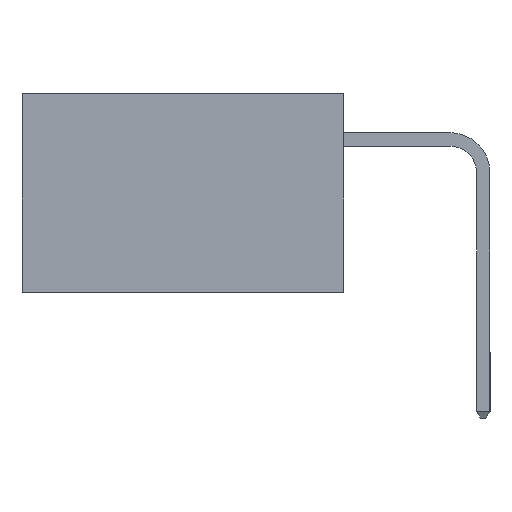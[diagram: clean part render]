
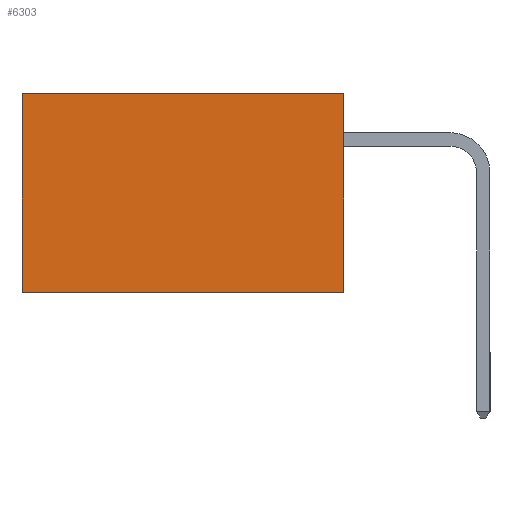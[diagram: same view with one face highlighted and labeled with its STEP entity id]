
A CAD part, left-side view. The second image highlights one B-rep face of the part: STEP entity #6303.
In plain terms, the highlighted planar face has unit normal (-1, 0, 0).
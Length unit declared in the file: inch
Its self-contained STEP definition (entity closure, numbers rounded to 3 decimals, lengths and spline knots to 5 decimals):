
#515 = VERTEX_POINT ( 'NONE', #8125 ) ;
#1023 = VECTOR ( 'NONE', #13386, 39.37008 ) ;
#2256 = VERTEX_POINT ( 'NONE', #5713 ) ;
#2532 = VERTEX_POINT ( 'NONE', #4521 ) ;
#2744 = FACE_OUTER_BOUND ( 'NONE', #3717, .T. ) ;
#2835 = ORIENTED_EDGE ( 'NONE', *, *, #6793, .T. ) ;
#2993 = ORIENTED_EDGE ( 'NONE', *, *, #3714, .T. ) ;
#3466 = EDGE_CURVE ( 'NONE', #515, #2256, #14345, .T. ) ;
#3616 = ORIENTED_EDGE ( 'NONE', *, *, #3466, .F. ) ;
#3714 = EDGE_CURVE ( 'NONE', #6412, #2256, #3801, .T. ) ;
#3717 = EDGE_LOOP ( 'NONE', ( #2993, #3616, #11207, #2835 ) ) ;
#3728 = DIRECTION ( 'NONE',  ( 0., 0., -1. ) ) ;
#3801 = LINE ( 'NONE', #6010, #5816 ) ;
#3802 = DIRECTION ( 'NONE',  ( 0., 0., -1. ) ) ;
#4031 = CARTESIAN_POINT ( 'NONE',  ( 0.2615, 0., -0.37 ) ) ;
#4169 = VECTOR ( 'NONE', #13963, 39.37008 ) ;
#4172 = LINE ( 'NONE', #9208, #4169 ) ;
#4521 = CARTESIAN_POINT ( 'NONE',  ( 0.2615, 0., 0. ) ) ;
#5713 = CARTESIAN_POINT ( 'NONE',  ( 0.2615, 0.6, -0.37 ) ) ;
#5816 = VECTOR ( 'NONE', #6088, 39.37008 ) ;
#6010 = CARTESIAN_POINT ( 'NONE',  ( 0.2615, 0.6, -0.37 ) ) ;
#6088 = DIRECTION ( 'NONE',  ( 0., 0., -1. ) ) ;
#6256 = CARTESIAN_POINT ( 'NONE',  ( 0.2615, 0., -0.37 ) ) ;
#6303 = ADVANCED_FACE ( 'NONE', ( #2744 ), #6404, .F. ) ;
#6328 = LINE ( 'NONE', #4031, #10316 ) ;
#6404 = PLANE ( 'NONE',  #9535 ) ;
#6412 = VERTEX_POINT ( 'NONE', #15394 ) ;
#6793 = EDGE_CURVE ( 'NONE', #2532, #6412, #4172, .T. ) ;
#8125 = CARTESIAN_POINT ( 'NONE',  ( 0.2615, 0., -0.37 ) ) ;
#9208 = CARTESIAN_POINT ( 'NONE',  ( 0.2615, 0., 0. ) ) ;
#9535 = AXIS2_PLACEMENT_3D ( 'NONE', #6256, #11197, #3728 ) ;
#10316 = VECTOR ( 'NONE', #3802, 39.37008 ) ;
#10764 = CARTESIAN_POINT ( 'NONE',  ( 0.2615, 0., -0.37 ) ) ;
#11197 = DIRECTION ( 'NONE',  ( 1., 0., 0. ) ) ;
#11207 = ORIENTED_EDGE ( 'NONE', *, *, #11904, .F. ) ;
#11904 = EDGE_CURVE ( 'NONE', #2532, #515, #6328, .T. ) ;
#13386 = DIRECTION ( 'NONE',  ( 0., 1., 0. ) ) ;
#13963 = DIRECTION ( 'NONE',  ( 0., 1., 0. ) ) ;
#14345 = LINE ( 'NONE', #10764, #1023 ) ;
#15394 = CARTESIAN_POINT ( 'NONE',  ( 0.2615, 0.6, 0. ) ) ;
